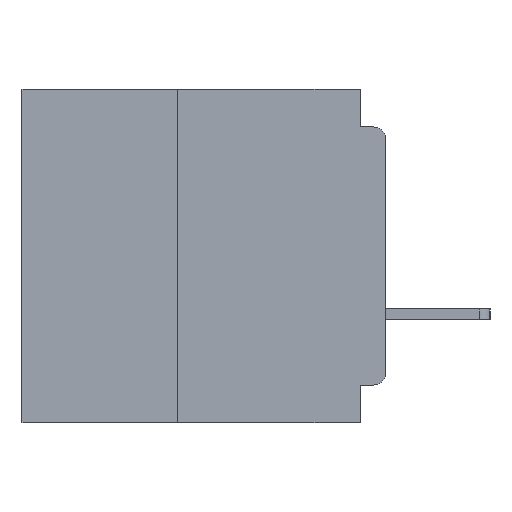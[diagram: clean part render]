
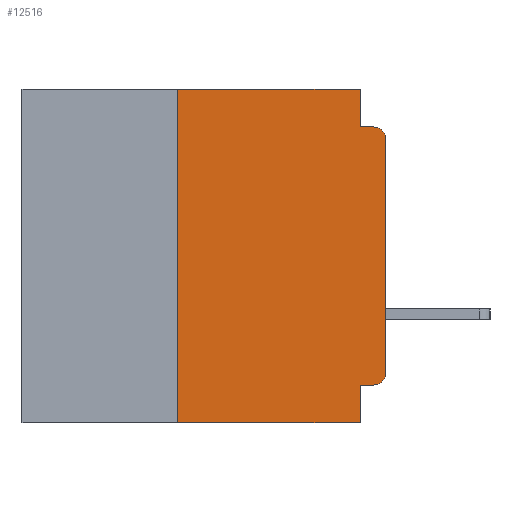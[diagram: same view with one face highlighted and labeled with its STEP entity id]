
A CAD part, left-side view. The second image highlights one B-rep face of the part: STEP entity #12516.
In plain terms, the highlighted planar face has unit normal (-1, 0, 0).
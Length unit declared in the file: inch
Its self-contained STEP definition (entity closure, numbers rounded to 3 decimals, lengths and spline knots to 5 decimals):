
#34 = LINE ( 'NONE', #1145, #41249 ) ;
#889 = EDGE_LOOP ( 'NONE', ( #15875, #41125, #23408, #46127, #44084, #2867, #1222, #35951, #8858, #25940 ) ) ;
#1145 = CARTESIAN_POINT ( 'NONE',  ( 0., 0.031, -0.4 ) ) ;
#1222 = ORIENTED_EDGE ( 'NONE', *, *, #10523, .T. ) ;
#1613 = CARTESIAN_POINT ( 'NONE',  ( 0., 0., -0.06 ) ) ;
#2867 = ORIENTED_EDGE ( 'NONE', *, *, #31766, .F. ) ;
#3754 = CARTESIAN_POINT ( 'NONE',  ( 0., 0.437, 0. ) ) ;
#4971 = EDGE_CURVE ( 'NONE', #6653, #19635, #36835, .T. ) ;
#5832 = CARTESIAN_POINT ( 'NONE',  ( 0., 0.015, -0.34 ) ) ;
#6407 = DIRECTION ( 'NONE',  ( 0., -1., 0. ) ) ;
#6653 = VERTEX_POINT ( 'NONE', #15860 ) ;
#7820 = PLANE ( 'NONE',  #12251 ) ;
#7964 = CARTESIAN_POINT ( 'NONE',  ( 0., 0., 0. ) ) ;
#8658 = VECTOR ( 'NONE', #6407, 39.37008 ) ;
#8858 = ORIENTED_EDGE ( 'NONE', *, *, #4971, .F. ) ;
#9414 = VERTEX_POINT ( 'NONE', #27608 ) ;
#9707 = CARTESIAN_POINT ( 'NONE',  ( 0., 0.25, -0.4 ) ) ;
#9864 = DIRECTION ( 'NONE',  ( 0., 0., -1. ) ) ;
#10233 = VECTOR ( 'NONE', #39293, 39.37008 ) ;
#10337 = EDGE_CURVE ( 'NONE', #19635, #34051, #34, .T. ) ;
#10523 = EDGE_CURVE ( 'NONE', #30157, #34051, #45195, .T. ) ;
#11555 = CARTESIAN_POINT ( 'NONE',  ( 0., 0., -0.045 ) ) ;
#11882 = DIRECTION ( 'NONE',  ( 0., 0., -1. ) ) ;
#12030 = LINE ( 'NONE', #7964, #44930 ) ;
#12251 = AXIS2_PLACEMENT_3D ( 'NONE', #3754, #35540, #11882 ) ;
#12516 = ADVANCED_FACE ( 'NONE', ( #30237 ), #7820, .F. ) ;
#13087 = CARTESIAN_POINT ( 'NONE',  ( 0., 0.25, -0.4 ) ) ;
#13580 = VECTOR ( 'NONE', #26789, 39.37008 ) ;
#14505 = DIRECTION ( 'NONE',  ( 0., 1., 0. ) ) ;
#15860 = CARTESIAN_POINT ( 'NONE',  ( 0., 0.015, -0.355 ) ) ;
#15875 = ORIENTED_EDGE ( 'NONE', *, *, #47674, .T. ) ;
#18131 = EDGE_CURVE ( 'NONE', #37869, #22724, #29980, .T. ) ;
#19635 = VERTEX_POINT ( 'NONE', #40862 ) ;
#21967 = DIRECTION ( 'NONE',  ( -1., 0., 0. ) ) ;
#22724 = VERTEX_POINT ( 'NONE', #23202 ) ;
#23202 = CARTESIAN_POINT ( 'NONE',  ( 0., 0.031, 0. ) ) ;
#23408 = ORIENTED_EDGE ( 'NONE', *, *, #23799, .F. ) ;
#23799 = EDGE_CURVE ( 'NONE', #35640, #30427, #40669, .T. ) ;
#23903 = VECTOR ( 'NONE', #36854, 39.37008 ) ;
#23912 = DIRECTION ( 'NONE',  ( 0., 0., 1. ) ) ;
#25194 = VECTOR ( 'NONE', #31433, 39.37008 ) ;
#25940 = ORIENTED_EDGE ( 'NONE', *, *, #30170, .T. ) ;
#26425 = LINE ( 'NONE', #13087, #23903 ) ;
#26789 = DIRECTION ( 'NONE',  ( 0., -1., 0. ) ) ;
#26959 = AXIS2_PLACEMENT_3D ( 'NONE', #5832, #33783, #9864 ) ;
#27608 = CARTESIAN_POINT ( 'NONE',  ( 0., 0., -0.34 ) ) ;
#29980 = LINE ( 'NONE', #30429, #8658 ) ;
#30130 = CIRCLE ( 'NONE', #35099, 0.015 ) ;
#30157 = VERTEX_POINT ( 'NONE', #9707 ) ;
#30170 = EDGE_CURVE ( 'NONE', #6653, #9414, #42604, .T. ) ;
#30237 = FACE_OUTER_BOUND ( 'NONE', #889, .T. ) ;
#30427 = VERTEX_POINT ( 'NONE', #31229 ) ;
#30429 = CARTESIAN_POINT ( 'NONE',  ( 0., 0.437, 0. ) ) ;
#31229 = CARTESIAN_POINT ( 'NONE',  ( 0., 0.015, -0.045 ) ) ;
#31433 = DIRECTION ( 'NONE',  ( 0., 0., -1. ) ) ;
#31766 = EDGE_CURVE ( 'NONE', #30157, #37869, #26425, .T. ) ;
#31975 = CARTESIAN_POINT ( 'NONE',  ( 0., 0.25, 0. ) ) ;
#33220 = DIRECTION ( 'NONE',  ( 0., 0., -1. ) ) ;
#33783 = DIRECTION ( 'NONE',  ( -1., 0., 0. ) ) ;
#34051 = VERTEX_POINT ( 'NONE', #38638 ) ;
#35099 = AXIS2_PLACEMENT_3D ( 'NONE', #45605, #21967, #49648 ) ;
#35305 = VERTEX_POINT ( 'NONE', #1613 ) ;
#35339 = CARTESIAN_POINT ( 'NONE',  ( 0., 0.031, 0. ) ) ;
#35540 = DIRECTION ( 'NONE',  ( 1., 0., 0. ) ) ;
#35640 = VERTEX_POINT ( 'NONE', #35687 ) ;
#35687 = CARTESIAN_POINT ( 'NONE',  ( 0., 0.031, -0.045 ) ) ;
#35951 = ORIENTED_EDGE ( 'NONE', *, *, #10337, .F. ) ;
#36835 = LINE ( 'NONE', #46203, #47392 ) ;
#36854 = DIRECTION ( 'NONE',  ( 0., 0., 1. ) ) ;
#37869 = VERTEX_POINT ( 'NONE', #31975 ) ;
#38638 = CARTESIAN_POINT ( 'NONE',  ( 0., 0.031, -0.4 ) ) ;
#39293 = DIRECTION ( 'NONE',  ( 0., -1., 0. ) ) ;
#40669 = LINE ( 'NONE', #11555, #10233 ) ;
#40862 = CARTESIAN_POINT ( 'NONE',  ( 0., 0.031, -0.355 ) ) ;
#41125 = ORIENTED_EDGE ( 'NONE', *, *, #45951, .T. ) ;
#41249 = VECTOR ( 'NONE', #33220, 39.37008 ) ;
#42604 = CIRCLE ( 'NONE', #26959, 0.015 ) ;
#44084 = ORIENTED_EDGE ( 'NONE', *, *, #18131, .F. ) ;
#44930 = VECTOR ( 'NONE', #23912, 39.37008 ) ;
#45195 = LINE ( 'NONE', #46434, #13580 ) ;
#45605 = CARTESIAN_POINT ( 'NONE',  ( 0., 0.015, -0.06 ) ) ;
#45951 = EDGE_CURVE ( 'NONE', #35305, #30427, #30130, .T. ) ;
#46127 = ORIENTED_EDGE ( 'NONE', *, *, #47617, .F. ) ;
#46203 = CARTESIAN_POINT ( 'NONE',  ( 0., 0., -0.355 ) ) ;
#46434 = CARTESIAN_POINT ( 'NONE',  ( 0., 0.437, -0.4 ) ) ;
#47392 = VECTOR ( 'NONE', #14505, 39.37008 ) ;
#47617 = EDGE_CURVE ( 'NONE', #22724, #35640, #49929, .T. ) ;
#47674 = EDGE_CURVE ( 'NONE', #9414, #35305, #12030, .T. ) ;
#49648 = DIRECTION ( 'NONE',  ( 0., 0., -1. ) ) ;
#49929 = LINE ( 'NONE', #35339, #25194 ) ;
